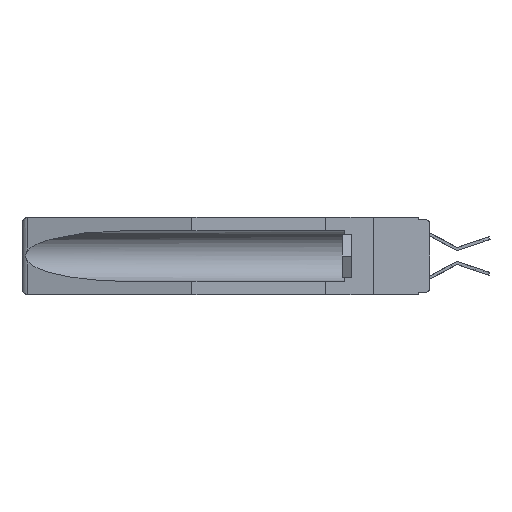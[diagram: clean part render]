
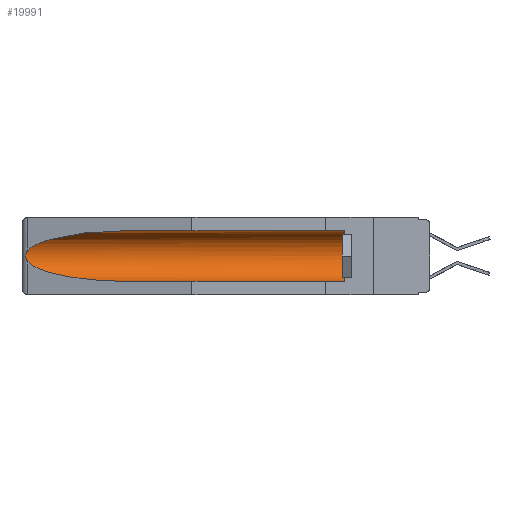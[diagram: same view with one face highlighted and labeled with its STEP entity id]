
A CAD part, left-side view. The second image highlights one B-rep face of the part: STEP entity #19991.
In plain terms, the highlighted cylindrical face has radius 2.857 mm (diameter 5.715 mm), a partial arc.
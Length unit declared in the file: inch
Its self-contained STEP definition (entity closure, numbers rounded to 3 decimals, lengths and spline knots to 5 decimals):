
#30 = CARTESIAN_POINT ( 'NONE',  ( 0.21114, 1.30732, -0.059 ) ) ;
#387 = CYLINDRICAL_SURFACE ( 'NONE', #5344, 0.1125 ) ;
#725 = CARTESIAN_POINT ( 'NONE',  ( 0.155, 1.07973, -0.059 ) ) ;
#739 = CARTESIAN_POINT ( 'NONE',  ( 0.25451, 1.48313, -0.24835 ) ) ;
#790 = VERTEX_POINT ( 'NONE', #725 ) ;
#864 = DIRECTION ( 'NONE',  ( 0., 0., 1. ) ) ;
#1605 = CARTESIAN_POINT ( 'NONE',  ( 0.26655, 1.53094, -0.18657 ) ) ;
#1811 = CARTESIAN_POINT ( 'NONE',  ( 0.26654, 1.53092, -0.15636 ) ) ;
#2474 = EDGE_CURVE ( 'NONE', #5011, #24531, #12272, .T. ) ;
#2895 = CARTESIAN_POINT ( 'NONE',  ( 0.26537, 1.52718, -0.19328 ) ) ;
#3094 = EDGE_CURVE ( 'NONE', #14498, #6584, #5074, .T. ) ;
#3549 = EDGE_LOOP ( 'NONE', ( #9782, #10824, #9035, #25481, #15501, #5979 ) ) ;
#3857 = CARTESIAN_POINT ( 'NONE',  ( 0.2675, 1.53308, -0.16763 ) ) ;
#4064 = CARTESIAN_POINT ( 'NONE',  ( 0.26597, 1.52961, -0.15275 ) ) ;
#5011 = VERTEX_POINT ( 'NONE', #21691 ) ;
#5074 = CIRCLE ( 'NONE', #28862, 0.1125 ) ;
#5344 = AXIS2_PLACEMENT_3D ( 'NONE', #14252, #7428, #864 ) ;
#5979 = ORIENTED_EDGE ( 'NONE', *, *, #21612, .T. ) ;
#5980 = CARTESIAN_POINT ( 'NONE',  ( 0.155, 0.126, -0.1715 ) ) ;
#6110 = CARTESIAN_POINT ( 'NONE',  ( 0.2675, 1.53308, -0.17534 ) ) ;
#6504 = CARTESIAN_POINT ( 'NONE',  ( 0.155, 0.126, -0.284 ) ) ;
#6584 = VERTEX_POINT ( 'NONE', #21523 ) ;
#7390 = CARTESIAN_POINT ( 'NONE',  ( 0.21114, 1.30732, -0.284 ) ) ;
#7428 = DIRECTION ( 'NONE',  ( 0., 1., 0. ) ) ;
#7981 =( BOUNDED_CURVE ( )  B_SPLINE_CURVE ( 3, ( #28865, #30, #22102, #9043 ),
 .UNSPECIFIED., .F., .F. ) 
 B_SPLINE_CURVE_WITH_KNOTS ( ( 4, 4 ),
 ( 4.71239, 6.08839 ),
 .UNSPECIFIED. ) 
 CURVE ( )  GEOMETRIC_REPRESENTATION_ITEM ( )  RATIONAL_B_SPLINE_CURVE ( ( 1., 0.848, 0.848, 1. ) ) 
 REPRESENTATION_ITEM ( '' )  );
#9035 = ORIENTED_EDGE ( 'NONE', *, *, #26786, .T. ) ;
#9043 = CARTESIAN_POINT ( 'NONE',  ( 0.26537, 1.52718, -0.14972 ) ) ;
#9782 = ORIENTED_EDGE ( 'NONE', *, *, #12769, .T. ) ;
#10008 = EDGE_CURVE ( 'NONE', #14498, #15421, #14830, .T. ) ;
#10346 = CARTESIAN_POINT ( 'NONE',  ( 0.155, -0.30754, -0.284 ) ) ;
#10533 = CARTESIAN_POINT ( 'NONE',  ( 0.2673, 1.5327, -0.16383 ) ) ;
#10824 = ORIENTED_EDGE ( 'NONE', *, *, #2474, .T. ) ;
#11265 = FACE_OUTER_BOUND ( 'NONE', #3549, .T. ) ;
#12272 = B_SPLINE_CURVE_WITH_KNOTS ( 'NONE', 3,
 ( #27796, #4064, #1811, #10533, #3857, #6110, #15104, #1605, #21828, #23923 ),
 .UNSPECIFIED., .F., .F.,
 ( 4, 2, 2, 2, 4 ),
 ( 0., 0.00029, 0.00058, 0.00087, 0.00117 ),
 .UNSPECIFIED. ) ;
#12632 = DIRECTION ( 'NONE',  ( 0., 0., 1. ) ) ;
#12769 = EDGE_CURVE ( 'NONE', #790, #5011, #7981, .T. ) ;
#13097 = CARTESIAN_POINT ( 'NONE',  ( 0.26537, 1.52718, -0.19328 ) ) ;
#14252 = CARTESIAN_POINT ( 'NONE',  ( 0.155, -0.30754, -0.1715 ) ) ;
#14459 = CARTESIAN_POINT ( 'NONE',  ( 0.155, 1.07973, -0.284 ) ) ;
#14498 = VERTEX_POINT ( 'NONE', #6504 ) ;
#14830 = LINE ( 'NONE', #10346, #25930 ) ;
#15104 = CARTESIAN_POINT ( 'NONE',  ( 0.2673, 1.53269, -0.17917 ) ) ;
#15421 = VERTEX_POINT ( 'NONE', #14459 ) ;
#15501 = ORIENTED_EDGE ( 'NONE', *, *, #3094, .T. ) ;
#19233 =( BOUNDED_CURVE ( )  B_SPLINE_CURVE ( 3, ( #2895, #739, #7390, #20265 ),
 .UNSPECIFIED., .F., .F. ) 
 B_SPLINE_CURVE_WITH_KNOTS ( ( 4, 4 ),
 ( 0.1948, 1.5708 ),
 .UNSPECIFIED. ) 
 CURVE ( )  GEOMETRIC_REPRESENTATION_ITEM ( )  RATIONAL_B_SPLINE_CURVE ( ( 1., 0.848, 0.848, 1. ) ) 
 REPRESENTATION_ITEM ( '' )  );
#19360 = DIRECTION ( 'NONE',  ( 0., -1., 0. ) ) ;
#19991 = ADVANCED_FACE ( 'NONE', ( #11265 ), #387, .F. ) ;
#20265 = CARTESIAN_POINT ( 'NONE',  ( 0.155, 1.07973, -0.284 ) ) ;
#21172 = DIRECTION ( 'NONE',  ( 0., 1., 0. ) ) ;
#21523 = CARTESIAN_POINT ( 'NONE',  ( 0.155, 0.126, -0.059 ) ) ;
#21564 = CARTESIAN_POINT ( 'NONE',  ( 0.155, -0.30754, -0.059 ) ) ;
#21612 = EDGE_CURVE ( 'NONE', #6584, #790, #27448, .T. ) ;
#21691 = CARTESIAN_POINT ( 'NONE',  ( 0.26537, 1.52718, -0.14972 ) ) ;
#21828 = CARTESIAN_POINT ( 'NONE',  ( 0.26597, 1.5296, -0.19026 ) ) ;
#22102 = CARTESIAN_POINT ( 'NONE',  ( 0.25451, 1.48313, -0.09465 ) ) ;
#23646 = VECTOR ( 'NONE', #23866, 39.37008 ) ;
#23866 = DIRECTION ( 'NONE',  ( 0., 1., 0. ) ) ;
#23923 = CARTESIAN_POINT ( 'NONE',  ( 0.26537, 1.52718, -0.19328 ) ) ;
#24531 = VERTEX_POINT ( 'NONE', #13097 ) ;
#25481 = ORIENTED_EDGE ( 'NONE', *, *, #10008, .F. ) ;
#25930 = VECTOR ( 'NONE', #21172, 39.37008 ) ;
#26786 = EDGE_CURVE ( 'NONE', #24531, #15421, #19233, .T. ) ;
#27448 = LINE ( 'NONE', #21564, #23646 ) ;
#27796 = CARTESIAN_POINT ( 'NONE',  ( 0.26537, 1.52718, -0.14972 ) ) ;
#28862 = AXIS2_PLACEMENT_3D ( 'NONE', #5980, #19360, #12632 ) ;
#28865 = CARTESIAN_POINT ( 'NONE',  ( 0.155, 1.07973, -0.059 ) ) ;
